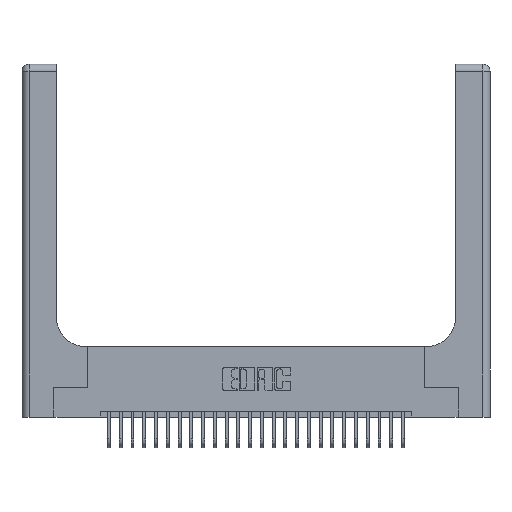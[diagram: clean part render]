
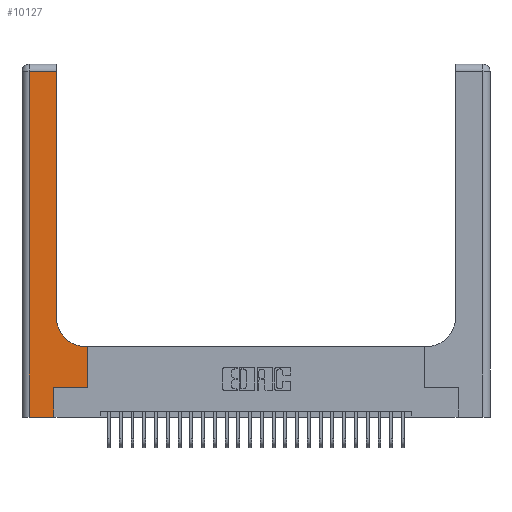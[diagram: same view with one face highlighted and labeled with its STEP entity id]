
A CAD part, top view. The second image highlights one B-rep face of the part: STEP entity #10127.
In plain terms, the highlighted planar face has unit normal (0, 0, 1).
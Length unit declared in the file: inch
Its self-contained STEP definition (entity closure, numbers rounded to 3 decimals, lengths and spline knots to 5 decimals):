
#119 = ORIENTED_EDGE ( 'NONE', *, *, #20157, .T. ) ;
#408 = VERTEX_POINT ( 'NONE', #10711 ) ;
#511 = LINE ( 'NONE', #2468, #14992 ) ;
#541 = EDGE_CURVE ( 'NONE', #19337, #9033, #20375, .T. ) ;
#601 = ORIENTED_EDGE ( 'NONE', *, *, #1358, .T. ) ;
#991 = CARTESIAN_POINT ( 'NONE',  ( 0.5415, 0.85, 0.37 ) ) ;
#1130 = VERTEX_POINT ( 'NONE', #2615 ) ;
#1227 = ORIENTED_EDGE ( 'NONE', *, *, #23819, .T. ) ;
#1358 = EDGE_CURVE ( 'NONE', #7305, #23983, #22417, .T. ) ;
#1555 = DIRECTION ( 'NONE',  ( 0., 0., -1. ) ) ;
#2139 = VECTOR ( 'NONE', #9107, 39.37008 ) ;
#2468 = CARTESIAN_POINT ( 'NONE',  ( 0.5585, 0.25, 0.37 ) ) ;
#2615 = CARTESIAN_POINT ( 'NONE',  ( 0.5415, 0.6, 0.37 ) ) ;
#2654 = CARTESIAN_POINT ( 'NONE',  ( 0.06, 3., 0.37 ) ) ;
#3936 = DIRECTION ( 'NONE',  ( -1., 0., 0. ) ) ;
#4622 = AXIS2_PLACEMENT_3D ( 'NONE', #991, #17187, #5584 ) ;
#4901 = VERTEX_POINT ( 'NONE', #21410 ) ;
#4979 = VERTEX_POINT ( 'NONE', #26167 ) ;
#5584 = DIRECTION ( 'NONE',  ( 1., 0., 0. ) ) ;
#5906 = EDGE_CURVE ( 'NONE', #16666, #7305, #23707, .T. ) ;
#6497 = VECTOR ( 'NONE', #10086, 39.37008 ) ;
#7033 = VECTOR ( 'NONE', #25638, 39.37008 ) ;
#7143 = EDGE_CURVE ( 'NONE', #408, #1130, #19057, .T. ) ;
#7248 = LINE ( 'NONE', #28429, #13295 ) ;
#7305 = VERTEX_POINT ( 'NONE', #24298 ) ;
#7468 = CIRCLE ( 'NONE', #4622, 0.25 ) ;
#7644 = ORIENTED_EDGE ( 'NONE', *, *, #541, .T. ) ;
#8411 = CARTESIAN_POINT ( 'NONE',  ( 0.06, 0., 0.37 ) ) ;
#9033 = VERTEX_POINT ( 'NONE', #27158 ) ;
#9107 = DIRECTION ( 'NONE',  ( 0., -1., 0. ) ) ;
#10086 = DIRECTION ( 'NONE',  ( -1., 0., 0. ) ) ;
#10127 = ADVANCED_FACE ( 'NONE', ( #21965 ), #28066, .F. ) ;
#10422 = CARTESIAN_POINT ( 'NONE',  ( 0.2915, 0.6, 0.37 ) ) ;
#10711 = CARTESIAN_POINT ( 'NONE',  ( 0.5585, 0.6, 0.37 ) ) ;
#12174 = ORIENTED_EDGE ( 'NONE', *, *, #5906, .T. ) ;
#12442 = ORIENTED_EDGE ( 'NONE', *, *, #25150, .T. ) ;
#13199 = VECTOR ( 'NONE', #19788, 39.37008 ) ;
#13295 = VECTOR ( 'NONE', #21864, 39.37008 ) ;
#14216 = LINE ( 'NONE', #2654, #2139 ) ;
#14992 = VECTOR ( 'NONE', #17987, 39.37008 ) ;
#16666 = VERTEX_POINT ( 'NONE', #8411 ) ;
#17108 = LINE ( 'NONE', #19786, #17837 ) ;
#17187 = DIRECTION ( 'NONE',  ( 0., 0., -1. ) ) ;
#17273 = ORIENTED_EDGE ( 'NONE', *, *, #22590, .T. ) ;
#17837 = VECTOR ( 'NONE', #24734, 39.37008 ) ;
#17886 = DIRECTION ( 'NONE',  ( -1., 0., 0. ) ) ;
#17987 = DIRECTION ( 'NONE',  ( 0., 1., 0. ) ) ;
#19057 = LINE ( 'NONE', #10422, #20116 ) ;
#19223 = CARTESIAN_POINT ( 'NONE',  ( 0., 2.94, 0.37 ) ) ;
#19337 = VERTEX_POINT ( 'NONE', #27890 ) ;
#19786 = CARTESIAN_POINT ( 'NONE',  ( 0.2915, 3., 0.37 ) ) ;
#19788 = DIRECTION ( 'NONE',  ( 0., 1., 0. ) ) ;
#20032 = ORIENTED_EDGE ( 'NONE', *, *, #21828, .T. ) ;
#20116 = VECTOR ( 'NONE', #17886, 39.37008 ) ;
#20157 = EDGE_CURVE ( 'NONE', #23983, #4979, #7248, .T. ) ;
#20375 = LINE ( 'NONE', #19223, #6497 ) ;
#20826 = CARTESIAN_POINT ( 'NONE',  ( 0.269, 0.25, 0.37 ) ) ;
#21410 = CARTESIAN_POINT ( 'NONE',  ( 0.2915, 0.85, 0.37 ) ) ;
#21453 = CARTESIAN_POINT ( 'NONE',  ( 0., 0., 0.37 ) ) ;
#21789 = CARTESIAN_POINT ( 'NONE',  ( 0., 3., 0.37 ) ) ;
#21828 = EDGE_CURVE ( 'NONE', #4901, #19337, #17108, .T. ) ;
#21864 = DIRECTION ( 'NONE',  ( 1., 0., 0. ) ) ;
#21943 = CARTESIAN_POINT ( 'NONE',  ( 0.269, 0., 0.37 ) ) ;
#21965 = FACE_OUTER_BOUND ( 'NONE', #29005, .T. ) ;
#22417 = LINE ( 'NONE', #21943, #13199 ) ;
#22590 = EDGE_CURVE ( 'NONE', #9033, #16666, #14216, .T. ) ;
#22698 = ORIENTED_EDGE ( 'NONE', *, *, #7143, .T. ) ;
#23707 = LINE ( 'NONE', #21453, #7033 ) ;
#23819 = EDGE_CURVE ( 'NONE', #4979, #408, #511, .T. ) ;
#23983 = VERTEX_POINT ( 'NONE', #20826 ) ;
#24298 = CARTESIAN_POINT ( 'NONE',  ( 0.269, 0., 0.37 ) ) ;
#24734 = DIRECTION ( 'NONE',  ( 0., 1., 0. ) ) ;
#25150 = EDGE_CURVE ( 'NONE', #1130, #4901, #7468, .T. ) ;
#25638 = DIRECTION ( 'NONE',  ( 1., 0., 0. ) ) ;
#26167 = CARTESIAN_POINT ( 'NONE',  ( 0.5585, 0.25, 0.37 ) ) ;
#26500 = AXIS2_PLACEMENT_3D ( 'NONE', #21789, #1555, #3936 ) ;
#27158 = CARTESIAN_POINT ( 'NONE',  ( 0.06, 2.94, 0.37 ) ) ;
#27890 = CARTESIAN_POINT ( 'NONE',  ( 0.2915, 2.94, 0.37 ) ) ;
#28066 = PLANE ( 'NONE',  #26500 ) ;
#28429 = CARTESIAN_POINT ( 'NONE',  ( 0.269, 0.25, 0.37 ) ) ;
#29005 = EDGE_LOOP ( 'NONE', ( #20032, #7644, #17273, #12174, #601, #119, #1227, #22698, #12442 ) ) ;
